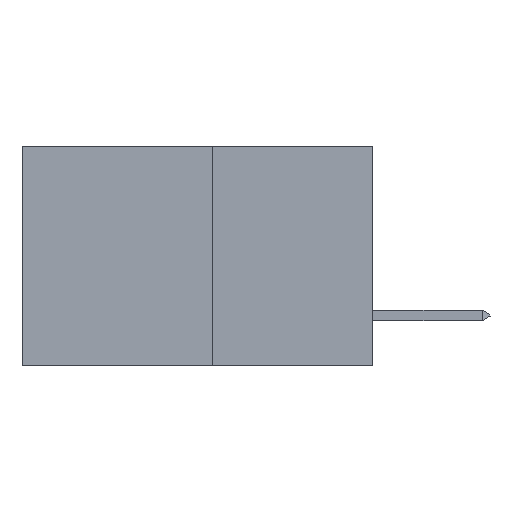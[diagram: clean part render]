
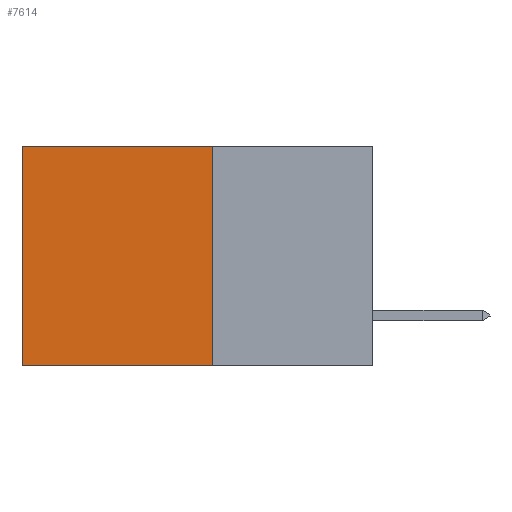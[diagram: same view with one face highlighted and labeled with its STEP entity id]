
A CAD part, left-side view. The second image highlights one B-rep face of the part: STEP entity #7614.
In plain terms, the highlighted planar face has unit normal (-1, 0, 0).
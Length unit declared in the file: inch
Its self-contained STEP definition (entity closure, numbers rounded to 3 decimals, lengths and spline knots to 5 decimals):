
#44 = VECTOR ( 'NONE', #2863, 39.37008 ) ;
#1761 = CARTESIAN_POINT ( 'NONE',  ( 0.277, 0.27, -0.37 ) ) ;
#1964 = EDGE_CURVE ( 'NONE', #10666, #12411, #9334, .T. ) ;
#2280 = ORIENTED_EDGE ( 'NONE', *, *, #2715, .T. ) ;
#2715 = EDGE_CURVE ( 'NONE', #3943, #10666, #9614, .T. ) ;
#2863 = DIRECTION ( 'NONE',  ( 0., 0., -1. ) ) ;
#3612 = CARTESIAN_POINT ( 'NONE',  ( 0.277, 0.59, 0. ) ) ;
#3943 = VERTEX_POINT ( 'NONE', #9689 ) ;
#4559 = CARTESIAN_POINT ( 'NONE',  ( 0.277, 0.59, -0.37 ) ) ;
#4694 = CARTESIAN_POINT ( 'NONE',  ( 0.277, 0.59, -0.37 ) ) ;
#5815 = DIRECTION ( 'NONE',  ( 0., 0., -1. ) ) ;
#6072 = DIRECTION ( 'NONE',  ( 0., 0., -1. ) ) ;
#6149 = EDGE_CURVE ( 'NONE', #6299, #12411, #10721, .T. ) ;
#6299 = VERTEX_POINT ( 'NONE', #9528 ) ;
#7031 = ORIENTED_EDGE ( 'NONE', *, *, #1964, .T. ) ;
#7079 = EDGE_LOOP ( 'NONE', ( #7031, #9664, #12569, #2280 ) ) ;
#7614 = ADVANCED_FACE ( 'NONE', ( #10998 ), #9779, .F. ) ;
#9102 = CARTESIAN_POINT ( 'NONE',  ( 0.277, 0.27, 0. ) ) ;
#9197 = DIRECTION ( 'NONE',  ( 0., 1., 0. ) ) ;
#9334 = LINE ( 'NONE', #4694, #11936 ) ;
#9461 = EDGE_CURVE ( 'NONE', #3943, #6299, #10976, .T. ) ;
#9498 = AXIS2_PLACEMENT_3D ( 'NONE', #10776, #11740, #5815 ) ;
#9528 = CARTESIAN_POINT ( 'NONE',  ( 0.277, 0.27, -0.37 ) ) ;
#9614 = LINE ( 'NONE', #9102, #11905 ) ;
#9664 = ORIENTED_EDGE ( 'NONE', *, *, #6149, .F. ) ;
#9689 = CARTESIAN_POINT ( 'NONE',  ( 0.277, 0.27, 0. ) ) ;
#9779 = PLANE ( 'NONE',  #9498 ) ;
#10666 = VERTEX_POINT ( 'NONE', #3612 ) ;
#10693 = DIRECTION ( 'NONE',  ( 0., 1., 0. ) ) ;
#10721 = LINE ( 'NONE', #10743, #12978 ) ;
#10743 = CARTESIAN_POINT ( 'NONE',  ( 0.277, 0.27, -0.37 ) ) ;
#10776 = CARTESIAN_POINT ( 'NONE',  ( 0.277, 0.27, -0.37 ) ) ;
#10976 = LINE ( 'NONE', #1761, #44 ) ;
#10998 = FACE_OUTER_BOUND ( 'NONE', #7079, .T. ) ;
#11740 = DIRECTION ( 'NONE',  ( 1., 0., 0. ) ) ;
#11905 = VECTOR ( 'NONE', #9197, 39.37008 ) ;
#11936 = VECTOR ( 'NONE', #6072, 39.37008 ) ;
#12411 = VERTEX_POINT ( 'NONE', #4559 ) ;
#12569 = ORIENTED_EDGE ( 'NONE', *, *, #9461, .F. ) ;
#12978 = VECTOR ( 'NONE', #10693, 39.37008 ) ;
